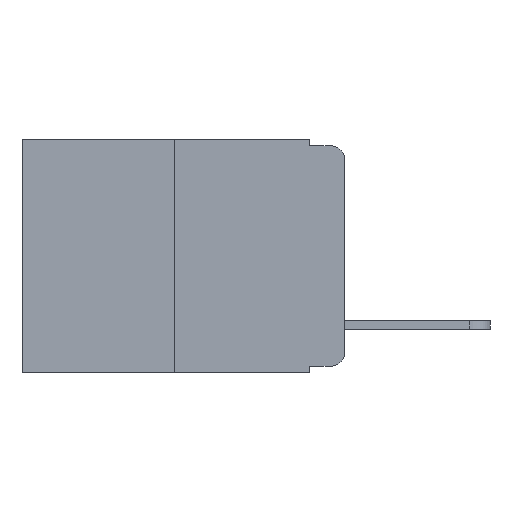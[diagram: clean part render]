
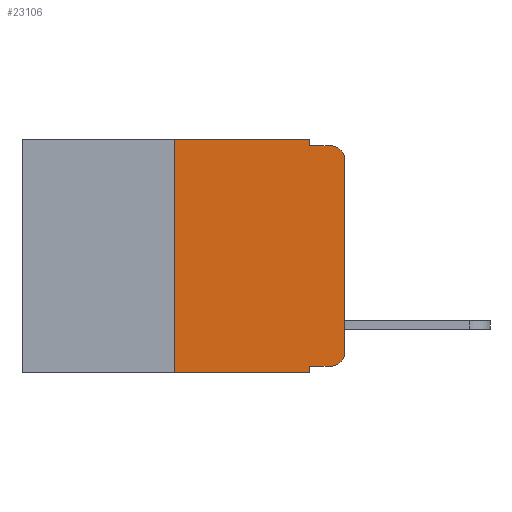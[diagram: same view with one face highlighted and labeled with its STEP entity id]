
A CAD part, left-side view. The second image highlights one B-rep face of the part: STEP entity #23106.
In plain terms, the highlighted planar face has unit normal (-1, 0, 0).
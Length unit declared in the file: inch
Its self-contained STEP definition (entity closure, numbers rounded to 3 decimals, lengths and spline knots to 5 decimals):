
#38 = LINE ( 'NONE', #3401, #12767 ) ;
#407 = EDGE_CURVE ( 'NONE', #1231, #15617, #12610, .T. ) ;
#1137 = LINE ( 'NONE', #26222, #22019 ) ;
#1231 = VERTEX_POINT ( 'NONE', #15483 ) ;
#1293 = FACE_OUTER_BOUND ( 'NONE', #26844, .T. ) ;
#1338 = CARTESIAN_POINT ( 'NONE',  ( 0., 0., -0.03 ) ) ;
#1974 = CARTESIAN_POINT ( 'NONE',  ( 0., 0.051, 0. ) ) ;
#1979 = ORIENTED_EDGE ( 'NONE', *, *, #4476, .F. ) ;
#2000 = ORIENTED_EDGE ( 'NONE', *, *, #17605, .F. ) ;
#2428 = VERTEX_POINT ( 'NONE', #19642 ) ;
#2524 = EDGE_CURVE ( 'NONE', #1231, #25907, #9245, .T. ) ;
#2723 = LINE ( 'NONE', #10923, #20665 ) ;
#2761 = CARTESIAN_POINT ( 'NONE',  ( 0., 0.02, -0.03 ) ) ;
#3401 = CARTESIAN_POINT ( 'NONE',  ( 0., 0.25, 0. ) ) ;
#4476 = EDGE_CURVE ( 'NONE', #19523, #8829, #16623, .T. ) ;
#5259 = CARTESIAN_POINT ( 'NONE',  ( 0., 0.02, -0.313 ) ) ;
#5310 = VECTOR ( 'NONE', #19797, 39.37008 ) ;
#5319 = DIRECTION ( 'NONE',  ( 0., -1., 0. ) ) ;
#5685 = VERTEX_POINT ( 'NONE', #1338 ) ;
#6200 = PLANE ( 'NONE',  #9255 ) ;
#6657 = CARTESIAN_POINT ( 'NONE',  ( 0., 0.051, 0. ) ) ;
#7198 = CARTESIAN_POINT ( 'NONE',  ( 0., 0.02, -0.333 ) ) ;
#7407 = EDGE_CURVE ( 'NONE', #24002, #15617, #23864, .T. ) ;
#7448 = DIRECTION ( 'NONE',  ( 0., 0., -1. ) ) ;
#7903 = EDGE_CURVE ( 'NONE', #13741, #5685, #9854, .T. ) ;
#8123 = DIRECTION ( 'NONE',  ( 0., 0., -1. ) ) ;
#8488 = ORIENTED_EDGE ( 'NONE', *, *, #7407, .T. ) ;
#8829 = VERTEX_POINT ( 'NONE', #1974 ) ;
#8985 = DIRECTION ( 'NONE',  ( -1., 0., 0. ) ) ;
#9036 = DIRECTION ( 'NONE',  ( 0., 0., 1. ) ) ;
#9087 = ORIENTED_EDGE ( 'NONE', *, *, #22307, .F. ) ;
#9245 = LINE ( 'NONE', #20263, #26132 ) ;
#9255 = AXIS2_PLACEMENT_3D ( 'NONE', #24840, #18610, #8123 ) ;
#9271 = CARTESIAN_POINT ( 'NONE',  ( 0., 0.25, -0.343 ) ) ;
#9854 = LINE ( 'NONE', #13133, #11811 ) ;
#10510 = CARTESIAN_POINT ( 'NONE',  ( 0., 0.25, 0. ) ) ;
#10779 = DIRECTION ( 'NONE',  ( 0., 0., -1. ) ) ;
#10923 = CARTESIAN_POINT ( 'NONE',  ( 0., 0.051, 0. ) ) ;
#11811 = VECTOR ( 'NONE', #9036, 39.37008 ) ;
#11993 = DIRECTION ( 'NONE',  ( 0., 0., 1. ) ) ;
#12031 = VERTEX_POINT ( 'NONE', #22642 ) ;
#12083 = VECTOR ( 'NONE', #5319, 39.37008 ) ;
#12116 = CIRCLE ( 'NONE', #14860, 0.02 ) ;
#12166 = ORIENTED_EDGE ( 'NONE', *, *, #7903, .T. ) ;
#12213 = ORIENTED_EDGE ( 'NONE', *, *, #2524, .T. ) ;
#12610 = LINE ( 'NONE', #6657, #25597 ) ;
#12767 = VECTOR ( 'NONE', #11993, 39.37008 ) ;
#13133 = CARTESIAN_POINT ( 'NONE',  ( 0., 0., 0. ) ) ;
#13189 = EDGE_CURVE ( 'NONE', #25907, #13741, #12116, .T. ) ;
#13741 = VERTEX_POINT ( 'NONE', #23498 ) ;
#13977 = DIRECTION ( 'NONE',  ( 0., -1., 0. ) ) ;
#14860 = AXIS2_PLACEMENT_3D ( 'NONE', #5259, #19732, #7448 ) ;
#15483 = CARTESIAN_POINT ( 'NONE',  ( 0., 0.051, -0.333 ) ) ;
#15617 = VERTEX_POINT ( 'NONE', #23958 ) ;
#16623 = LINE ( 'NONE', #25792, #12083 ) ;
#17023 = DIRECTION ( 'NONE',  ( 0., 0., -1. ) ) ;
#17605 = EDGE_CURVE ( 'NONE', #8829, #2428, #2723, .T. ) ;
#18610 = DIRECTION ( 'NONE',  ( 1., 0., 0. ) ) ;
#19031 = DIRECTION ( 'NONE',  ( 0., 0., -1. ) ) ;
#19274 = ORIENTED_EDGE ( 'NONE', *, *, #407, .F. ) ;
#19335 = EDGE_CURVE ( 'NONE', #2428, #12031, #1137, .T. ) ;
#19523 = VERTEX_POINT ( 'NONE', #10510 ) ;
#19642 = CARTESIAN_POINT ( 'NONE',  ( 0., 0.051, -0.01 ) ) ;
#19732 = DIRECTION ( 'NONE',  ( -1., 0., 0. ) ) ;
#19797 = DIRECTION ( 'NONE',  ( 0., -1., 0. ) ) ;
#19933 = ORIENTED_EDGE ( 'NONE', *, *, #13189, .T. ) ;
#20140 = CIRCLE ( 'NONE', #24567, 0.02 ) ;
#20263 = CARTESIAN_POINT ( 'NONE',  ( 0., 0.051, -0.333 ) ) ;
#20665 = VECTOR ( 'NONE', #19031, 39.37008 ) ;
#22019 = VECTOR ( 'NONE', #13977, 39.37008 ) ;
#22307 = EDGE_CURVE ( 'NONE', #24002, #19523, #38, .T. ) ;
#22642 = CARTESIAN_POINT ( 'NONE',  ( 0., 0.02, -0.01 ) ) ;
#23106 = ADVANCED_FACE ( 'NONE', ( #1293 ), #6200, .F. ) ;
#23498 = CARTESIAN_POINT ( 'NONE',  ( 0., 0., -0.313 ) ) ;
#23864 = LINE ( 'NONE', #24327, #5310 ) ;
#23935 = EDGE_CURVE ( 'NONE', #5685, #12031, #20140, .T. ) ;
#23958 = CARTESIAN_POINT ( 'NONE',  ( 0., 0.051, -0.343 ) ) ;
#24002 = VERTEX_POINT ( 'NONE', #9271 ) ;
#24175 = DIRECTION ( 'NONE',  ( 0., -1., 0. ) ) ;
#24197 = ORIENTED_EDGE ( 'NONE', *, *, #23935, .T. ) ;
#24327 = CARTESIAN_POINT ( 'NONE',  ( 0., 0.473, -0.343 ) ) ;
#24567 = AXIS2_PLACEMENT_3D ( 'NONE', #2761, #8985, #17023 ) ;
#24840 = CARTESIAN_POINT ( 'NONE',  ( 0., 0.473, 0. ) ) ;
#25597 = VECTOR ( 'NONE', #10779, 39.37008 ) ;
#25792 = CARTESIAN_POINT ( 'NONE',  ( 0., 0.473, 0. ) ) ;
#25907 = VERTEX_POINT ( 'NONE', #7198 ) ;
#26132 = VECTOR ( 'NONE', #24175, 39.37008 ) ;
#26222 = CARTESIAN_POINT ( 'NONE',  ( 0., 0.051, -0.01 ) ) ;
#26356 = ORIENTED_EDGE ( 'NONE', *, *, #19335, .F. ) ;
#26844 = EDGE_LOOP ( 'NONE', ( #12166, #24197, #26356, #2000, #1979, #9087, #8488, #19274, #12213, #19933 ) ) ;
